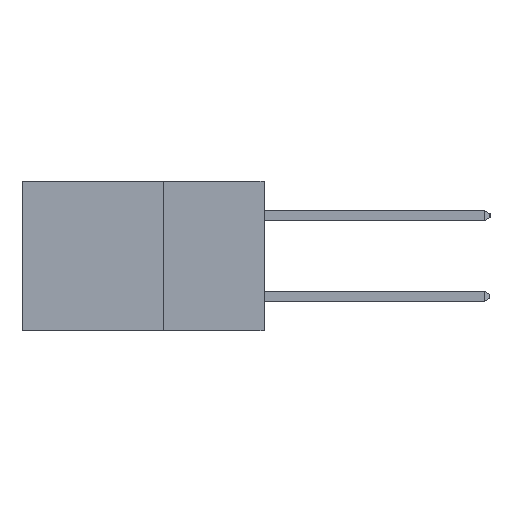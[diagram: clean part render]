
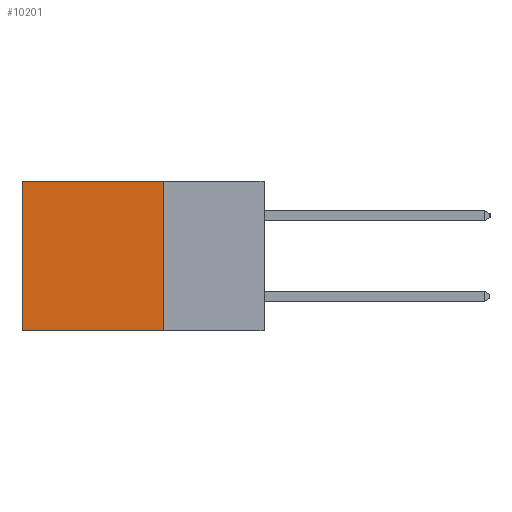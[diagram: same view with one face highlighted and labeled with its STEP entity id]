
A CAD part, left-side view. The second image highlights one B-rep face of the part: STEP entity #10201.
In plain terms, the highlighted planar face has unit normal (-1, 0, 0).
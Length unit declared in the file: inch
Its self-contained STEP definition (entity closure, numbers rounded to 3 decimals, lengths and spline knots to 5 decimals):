
#190 = VERTEX_POINT ( 'NONE', #6802 ) ;
#583 = CARTESIAN_POINT ( 'NONE',  ( 0.2615, 0.25, -0.37 ) ) ;
#716 = DIRECTION ( 'NONE',  ( 0., 0., -1. ) ) ;
#722 = LINE ( 'NONE', #6139, #8245 ) ;
#888 = VECTOR ( 'NONE', #7214, 39.37008 ) ;
#2224 = EDGE_CURVE ( 'NONE', #13057, #12854, #4476, .T. ) ;
#2809 = LINE ( 'NONE', #7900, #4780 ) ;
#2958 = FACE_OUTER_BOUND ( 'NONE', #4644, .T. ) ;
#4109 = LINE ( 'NONE', #6079, #888 ) ;
#4407 = CARTESIAN_POINT ( 'NONE',  ( 0.2615, 0.6, -0.37 ) ) ;
#4436 = CARTESIAN_POINT ( 'NONE',  ( 0.2615, 0.6, 0. ) ) ;
#4476 = LINE ( 'NONE', #4407, #7492 ) ;
#4644 = EDGE_LOOP ( 'NONE', ( #7711, #11636, #8712, #5806 ) ) ;
#4780 = VECTOR ( 'NONE', #716, 39.37008 ) ;
#5118 = CARTESIAN_POINT ( 'NONE',  ( 0.2615, 0.6, -0.37 ) ) ;
#5806 = ORIENTED_EDGE ( 'NONE', *, *, #8849, .T. ) ;
#6079 = CARTESIAN_POINT ( 'NONE',  ( 0.2615, 0.25, -0.37 ) ) ;
#6139 = CARTESIAN_POINT ( 'NONE',  ( 0.2615, 0.25, 0. ) ) ;
#6141 = DIRECTION ( 'NONE',  ( 1., 0., 0. ) ) ;
#6802 = CARTESIAN_POINT ( 'NONE',  ( 0.2615, 0.25, 0. ) ) ;
#7214 = DIRECTION ( 'NONE',  ( 0., 1., 0. ) ) ;
#7492 = VECTOR ( 'NONE', #12779, 39.37008 ) ;
#7711 = ORIENTED_EDGE ( 'NONE', *, *, #2224, .T. ) ;
#7874 = EDGE_CURVE ( 'NONE', #190, #12773, #2809, .T. ) ;
#7900 = CARTESIAN_POINT ( 'NONE',  ( 0.2615, 0.25, -0.37 ) ) ;
#8245 = VECTOR ( 'NONE', #9406, 39.37008 ) ;
#8712 = ORIENTED_EDGE ( 'NONE', *, *, #7874, .F. ) ;
#8849 = EDGE_CURVE ( 'NONE', #190, #13057, #722, .T. ) ;
#8868 = EDGE_CURVE ( 'NONE', #12773, #12854, #4109, .T. ) ;
#9040 = DIRECTION ( 'NONE',  ( 0., 0., -1. ) ) ;
#9302 = PLANE ( 'NONE',  #12795 ) ;
#9406 = DIRECTION ( 'NONE',  ( 0., 1., 0. ) ) ;
#10201 = ADVANCED_FACE ( 'NONE', ( #2958 ), #9302, .F. ) ;
#11636 = ORIENTED_EDGE ( 'NONE', *, *, #8868, .F. ) ;
#12143 = CARTESIAN_POINT ( 'NONE',  ( 0.2615, 0.25, -0.37 ) ) ;
#12773 = VERTEX_POINT ( 'NONE', #583 ) ;
#12779 = DIRECTION ( 'NONE',  ( 0., 0., -1. ) ) ;
#12795 = AXIS2_PLACEMENT_3D ( 'NONE', #12143, #6141, #9040 ) ;
#12854 = VERTEX_POINT ( 'NONE', #5118 ) ;
#13057 = VERTEX_POINT ( 'NONE', #4436 ) ;
